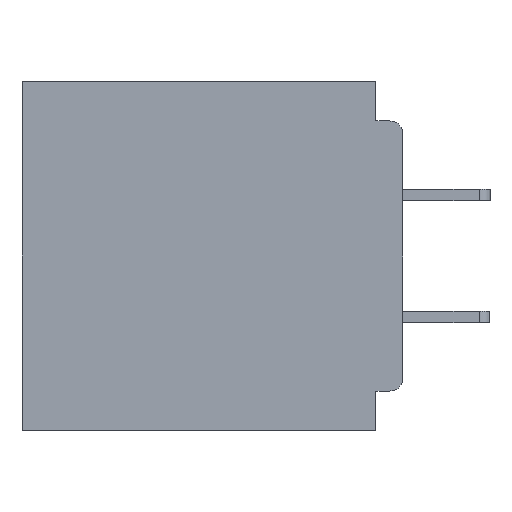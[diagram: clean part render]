
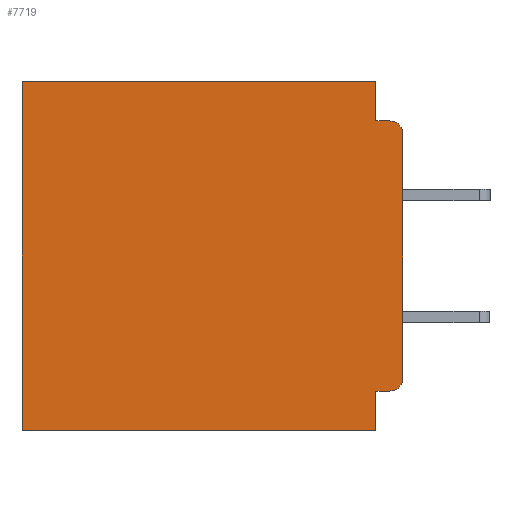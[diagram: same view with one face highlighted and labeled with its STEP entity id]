
A CAD part, left-side view. The second image highlights one B-rep face of the part: STEP entity #7719.
In plain terms, the highlighted planar face has unit normal (-1, 0, 0).
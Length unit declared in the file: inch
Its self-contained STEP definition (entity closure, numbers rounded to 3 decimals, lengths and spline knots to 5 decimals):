
#692 = DIRECTION ( 'NONE',  ( 0., 0., -1. ) ) ;
#1206 = CARTESIAN_POINT ( 'NONE',  ( 0.3, 0.015, -0.045 ) ) ;
#1291 = ORIENTED_EDGE ( 'NONE', *, *, #9454, .F. ) ;
#1299 = VECTOR ( 'NONE', #5620, 39.37008 ) ;
#2160 = ORIENTED_EDGE ( 'NONE', *, *, #19707, .F. ) ;
#2164 = CARTESIAN_POINT ( 'NONE',  ( 0.3, 0.015, -0.34 ) ) ;
#3592 = ORIENTED_EDGE ( 'NONE', *, *, #17959, .T. ) ;
#4373 = LINE ( 'NONE', #6470, #19445 ) ;
#4790 = VERTEX_POINT ( 'NONE', #15499 ) ;
#4935 = VERTEX_POINT ( 'NONE', #12341 ) ;
#5154 = VECTOR ( 'NONE', #24020, 39.37008 ) ;
#5185 = CARTESIAN_POINT ( 'NONE',  ( 0.3, 0., -0.355 ) ) ;
#5208 = DIRECTION ( 'NONE',  ( 0., 0., -1. ) ) ;
#5324 = CARTESIAN_POINT ( 'NONE',  ( 0.3, 0., -0.4 ) ) ;
#5448 = DIRECTION ( 'NONE',  ( 0., 1., 0. ) ) ;
#5620 = DIRECTION ( 'NONE',  ( 0., 0., -1. ) ) ;
#5637 = ORIENTED_EDGE ( 'NONE', *, *, #19217, .F. ) ;
#5790 = VERTEX_POINT ( 'NONE', #30556 ) ;
#6470 = CARTESIAN_POINT ( 'NONE',  ( 0.3, 0.437, -0.4 ) ) ;
#6586 = EDGE_CURVE ( 'NONE', #4935, #8374, #4373, .T. ) ;
#7671 = DIRECTION ( 'NONE',  ( 0., 0., -1. ) ) ;
#7719 = ADVANCED_FACE ( 'NONE', ( #12768 ), #8901, .F. ) ;
#7977 = ORIENTED_EDGE ( 'NONE', *, *, #18736, .F. ) ;
#8374 = VERTEX_POINT ( 'NONE', #20770 ) ;
#8901 = PLANE ( 'NONE',  #26602 ) ;
#9312 = LINE ( 'NONE', #5185, #16364 ) ;
#9454 = EDGE_CURVE ( 'NONE', #28893, #22887, #29869, .T. ) ;
#9876 = CARTESIAN_POINT ( 'NONE',  ( 0.3, 0.031, -0.4 ) ) ;
#10695 = CARTESIAN_POINT ( 'NONE',  ( 0.3, 0.031, 0. ) ) ;
#11408 = EDGE_CURVE ( 'NONE', #5790, #33021, #31618, .T. ) ;
#12197 = CARTESIAN_POINT ( 'NONE',  ( 0.3, 0., -0.4 ) ) ;
#12341 = CARTESIAN_POINT ( 'NONE',  ( 0.3, 0.437, 0. ) ) ;
#12768 = FACE_OUTER_BOUND ( 'NONE', #28657, .T. ) ;
#12888 = ORIENTED_EDGE ( 'NONE', *, *, #28653, .F. ) ;
#14010 = VECTOR ( 'NONE', #22423, 39.37008 ) ;
#14097 = AXIS2_PLACEMENT_3D ( 'NONE', #2164, #23211, #5208 ) ;
#14270 = CARTESIAN_POINT ( 'NONE',  ( 0.3, 0.031, -0.355 ) ) ;
#14705 = LINE ( 'NONE', #5324, #37478 ) ;
#14904 = VECTOR ( 'NONE', #38576, 39.37008 ) ;
#14935 = CARTESIAN_POINT ( 'NONE',  ( 0.3, 0., -0.34 ) ) ;
#14951 = CARTESIAN_POINT ( 'NONE',  ( 0.3, 0., -0.4 ) ) ;
#15088 = ORIENTED_EDGE ( 'NONE', *, *, #34687, .F. ) ;
#15499 = CARTESIAN_POINT ( 'NONE',  ( 0.3, 0.031, 0. ) ) ;
#16364 = VECTOR ( 'NONE', #20156, 39.37008 ) ;
#16416 = CARTESIAN_POINT ( 'NONE',  ( 0.3, 0., -0.045 ) ) ;
#16577 = VERTEX_POINT ( 'NONE', #17784 ) ;
#17334 = LINE ( 'NONE', #12197, #1299 ) ;
#17784 = CARTESIAN_POINT ( 'NONE',  ( 0.3, 0., -0.06 ) ) ;
#17938 = DIRECTION ( 'NONE',  ( 0., 0., -1. ) ) ;
#17959 = EDGE_CURVE ( 'NONE', #16577, #22887, #22005, .T. ) ;
#18719 = DIRECTION ( 'NONE',  ( -1., 0., 0. ) ) ;
#18736 = EDGE_CURVE ( 'NONE', #16577, #33021, #17334, .T. ) ;
#19182 = ORIENTED_EDGE ( 'NONE', *, *, #11408, .T. ) ;
#19217 = EDGE_CURVE ( 'NONE', #5790, #34666, #9312, .T. ) ;
#19445 = VECTOR ( 'NONE', #30369, 39.37008 ) ;
#19524 = ORIENTED_EDGE ( 'NONE', *, *, #21942, .T. ) ;
#19707 = EDGE_CURVE ( 'NONE', #4790, #28893, #38130, .T. ) ;
#20156 = DIRECTION ( 'NONE',  ( 0., 1., 0. ) ) ;
#20770 = CARTESIAN_POINT ( 'NONE',  ( 0.3, 0.437, -0.4 ) ) ;
#21000 = CARTESIAN_POINT ( 'NONE',  ( 0.3, 0., 0. ) ) ;
#21942 = EDGE_CURVE ( 'NONE', #4790, #4935, #29025, .T. ) ;
#22005 = CIRCLE ( 'NONE', #34460, 0.015 ) ;
#22423 = DIRECTION ( 'NONE',  ( 0., -1., 0. ) ) ;
#22844 = LINE ( 'NONE', #26694, #14904 ) ;
#22887 = VERTEX_POINT ( 'NONE', #1206 ) ;
#23211 = DIRECTION ( 'NONE',  ( -1., 0., 0. ) ) ;
#24020 = DIRECTION ( 'NONE',  ( 0., 1., 0. ) ) ;
#25597 = ORIENTED_EDGE ( 'NONE', *, *, #6586, .T. ) ;
#26602 = AXIS2_PLACEMENT_3D ( 'NONE', #14951, #35755, #17938 ) ;
#26694 = CARTESIAN_POINT ( 'NONE',  ( 0.3, 0.031, -0.4 ) ) ;
#28653 = EDGE_CURVE ( 'NONE', #34666, #37686, #22844, .T. ) ;
#28657 = EDGE_LOOP ( 'NONE', ( #7977, #3592, #1291, #2160, #19524, #25597, #15088, #12888, #5637, #19182 ) ) ;
#28893 = VERTEX_POINT ( 'NONE', #30674 ) ;
#29025 = LINE ( 'NONE', #21000, #5154 ) ;
#29869 = LINE ( 'NONE', #16416, #14010 ) ;
#30271 = VECTOR ( 'NONE', #7671, 39.37008 ) ;
#30369 = DIRECTION ( 'NONE',  ( 0., 0., -1. ) ) ;
#30556 = CARTESIAN_POINT ( 'NONE',  ( 0.3, 0.015, -0.355 ) ) ;
#30674 = CARTESIAN_POINT ( 'NONE',  ( 0.3, 0.031, -0.045 ) ) ;
#31618 = CIRCLE ( 'NONE', #14097, 0.015 ) ;
#33021 = VERTEX_POINT ( 'NONE', #14935 ) ;
#34460 = AXIS2_PLACEMENT_3D ( 'NONE', #36541, #18719, #692 ) ;
#34666 = VERTEX_POINT ( 'NONE', #14270 ) ;
#34687 = EDGE_CURVE ( 'NONE', #37686, #8374, #14705, .T. ) ;
#35755 = DIRECTION ( 'NONE',  ( 1., 0., 0. ) ) ;
#36541 = CARTESIAN_POINT ( 'NONE',  ( 0.3, 0.015, -0.06 ) ) ;
#37478 = VECTOR ( 'NONE', #5448, 39.37008 ) ;
#37686 = VERTEX_POINT ( 'NONE', #9876 ) ;
#38130 = LINE ( 'NONE', #10695, #30271 ) ;
#38576 = DIRECTION ( 'NONE',  ( 0., 0., -1. ) ) ;
